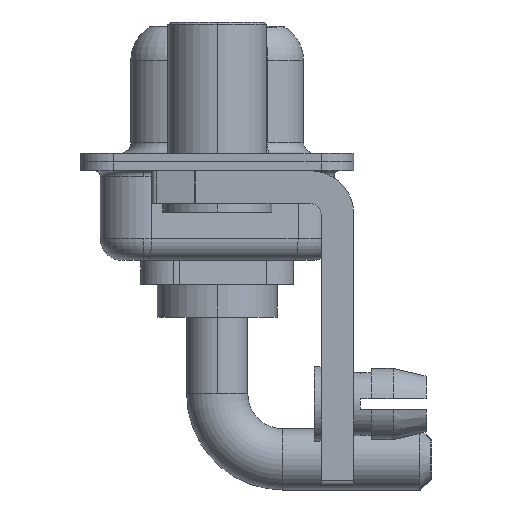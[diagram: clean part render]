
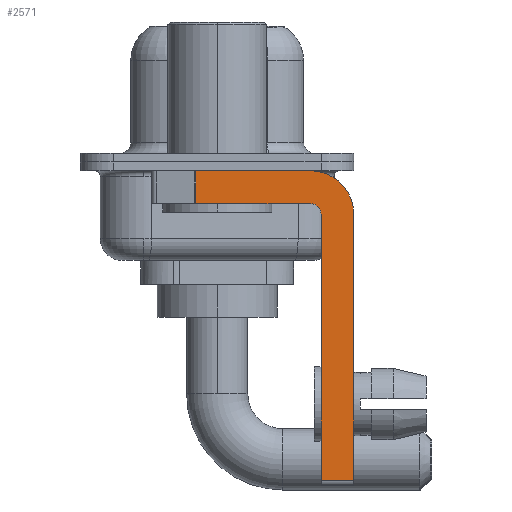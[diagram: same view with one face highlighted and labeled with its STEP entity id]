
A CAD part, left-side view. The second image highlights one B-rep face of the part: STEP entity #2571.
In plain terms, the highlighted planar face has unit normal (-1, 0, 0).
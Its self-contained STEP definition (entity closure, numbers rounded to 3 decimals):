
#8 = EDGE_CURVE ( 'NONE', #11833, #8925, #10936, .T. ) ;
#270 = ORIENTED_EDGE ( 'NONE', *, *, #3088, .T. ) ;
#495 = VECTOR ( 'NONE', #10711, 1000. ) ;
#551 = CARTESIAN_POINT ( 'NONE',  ( -2.9, -4.75, -14.8 ) ) ;
#1016 = AXIS2_PLACEMENT_3D ( 'NONE', #15161, #17780, #2743 ) ;
#1259 = AXIS2_PLACEMENT_3D ( 'NONE', #3979, #17837, #14841 ) ;
#1938 = CARTESIAN_POINT ( 'NONE',  ( -2.9, 0.978, -1.9 ) ) ;
#2002 = VECTOR ( 'NONE', #9836, 1000. ) ;
#2188 = EDGE_CURVE ( 'NONE', #5790, #9103, #14900, .T. ) ;
#2571 = ADVANCED_FACE ( 'NONE', ( #14587 ), #3723, .F. ) ;
#2743 = DIRECTION ( 'NONE',  ( 0., 0., -1. ) ) ;
#2766 = CARTESIAN_POINT ( 'NONE',  ( -2.9, 0.978, -1.9 ) ) ;
#2880 = ORIENTED_EDGE ( 'NONE', *, *, #8, .T. ) ;
#2889 = VECTOR ( 'NONE', #16791, 1000. ) ;
#3088 = EDGE_CURVE ( 'NONE', #12082, #17735, #5502, .T. ) ;
#3380 = ORIENTED_EDGE ( 'NONE', *, *, #2188, .F. ) ;
#3723 = PLANE ( 'NONE',  #8751 ) ;
#3870 = CIRCLE ( 'NONE', #1259, 0.5 ) ;
#3979 = CARTESIAN_POINT ( 'NONE',  ( -2.9, -4.25, -2.4 ) ) ;
#4221 = DIRECTION ( 'NONE',  ( 0., 0., -1. ) ) ;
#4490 = EDGE_CURVE ( 'NONE', #13810, #11897, #3870, .T. ) ;
#5165 = ORIENTED_EDGE ( 'NONE', *, *, #4490, .F. ) ;
#5502 = LINE ( 'NONE', #2766, #15996 ) ;
#5790 = VERTEX_POINT ( 'NONE', #6517 ) ;
#6301 = CARTESIAN_POINT ( 'NONE',  ( -2.9, -4.75, -14.55 ) ) ;
#6471 = ORIENTED_EDGE ( 'NONE', *, *, #12904, .F. ) ;
#6517 = CARTESIAN_POINT ( 'NONE',  ( -2.9, -4.25, -0.4 ) ) ;
#6933 = CARTESIAN_POINT ( 'NONE',  ( -2.9, -4.25, -14.55 ) ) ;
#7136 = ORIENTED_EDGE ( 'NONE', *, *, #9613, .F. ) ;
#7945 = LINE ( 'NONE', #14921, #8351 ) ;
#7974 = ORIENTED_EDGE ( 'NONE', *, *, #14356, .F. ) ;
#8351 = VECTOR ( 'NONE', #12225, 1000. ) ;
#8751 = AXIS2_PLACEMENT_3D ( 'NONE', #9252, #15782, #14774 ) ;
#8925 = VERTEX_POINT ( 'NONE', #14271 ) ;
#9103 = VERTEX_POINT ( 'NONE', #14860 ) ;
#9252 = CARTESIAN_POINT ( 'NONE',  ( -2.9, -4.25, -2.4 ) ) ;
#9613 = EDGE_CURVE ( 'NONE', #11897, #17735, #12234, .T. ) ;
#9836 = DIRECTION ( 'NONE',  ( 0., -1., 0. ) ) ;
#9930 = CARTESIAN_POINT ( 'NONE',  ( -2.9, 0.978, -0.4 ) ) ;
#10156 = DIRECTION ( 'NONE',  ( 0., 0., -1. ) ) ;
#10711 = DIRECTION ( 'NONE',  ( 0., 1., 0. ) ) ;
#10936 = LINE ( 'NONE', #6933, #2002 ) ;
#10983 = CARTESIAN_POINT ( 'NONE',  ( -2.9, -4.25, -1.9 ) ) ;
#11107 = EDGE_CURVE ( 'NONE', #9103, #8925, #11610, .T. ) ;
#11456 = LINE ( 'NONE', #551, #2889 ) ;
#11610 = LINE ( 'NONE', #11786, #13285 ) ;
#11786 = CARTESIAN_POINT ( 'NONE',  ( -2.9, -6.25, -2.4 ) ) ;
#11833 = VERTEX_POINT ( 'NONE', #6301 ) ;
#11897 = VERTEX_POINT ( 'NONE', #13553 ) ;
#12082 = VERTEX_POINT ( 'NONE', #9930 ) ;
#12225 = DIRECTION ( 'NONE',  ( 0., -1., 0. ) ) ;
#12234 = LINE ( 'NONE', #10983, #495 ) ;
#12904 = EDGE_CURVE ( 'NONE', #12082, #5790, #7945, .T. ) ;
#13285 = VECTOR ( 'NONE', #10156, 1000. ) ;
#13553 = CARTESIAN_POINT ( 'NONE',  ( -2.9, -4.25, -1.9 ) ) ;
#13810 = VERTEX_POINT ( 'NONE', #16896 ) ;
#14271 = CARTESIAN_POINT ( 'NONE',  ( -2.9, -6.25, -14.55 ) ) ;
#14356 = EDGE_CURVE ( 'NONE', #11833, #13810, #11456, .T. ) ;
#14587 = FACE_OUTER_BOUND ( 'NONE', #15756, .T. ) ;
#14774 = DIRECTION ( 'NONE',  ( 0., 0., -1. ) ) ;
#14841 = DIRECTION ( 'NONE',  ( 0., 0., 1. ) ) ;
#14860 = CARTESIAN_POINT ( 'NONE',  ( -2.9, -6.25, -2.4 ) ) ;
#14900 = CIRCLE ( 'NONE', #1016, 2. ) ;
#14921 = CARTESIAN_POINT ( 'NONE',  ( -2.9, 3., -0.4 ) ) ;
#15161 = CARTESIAN_POINT ( 'NONE',  ( -2.9, -4.25, -2.4 ) ) ;
#15756 = EDGE_LOOP ( 'NONE', ( #6471, #270, #7136, #5165, #7974, #2880, #17086, #3380 ) ) ;
#15782 = DIRECTION ( 'NONE',  ( 1., 0., 0. ) ) ;
#15996 = VECTOR ( 'NONE', #4221, 1000. ) ;
#16791 = DIRECTION ( 'NONE',  ( 0., 0., 1. ) ) ;
#16896 = CARTESIAN_POINT ( 'NONE',  ( -2.9, -4.75, -2.4 ) ) ;
#17086 = ORIENTED_EDGE ( 'NONE', *, *, #11107, .F. ) ;
#17735 = VERTEX_POINT ( 'NONE', #1938 ) ;
#17780 = DIRECTION ( 'NONE',  ( 1., 0., 0. ) ) ;
#17837 = DIRECTION ( 'NONE',  ( -1., 0., 0. ) ) ;
